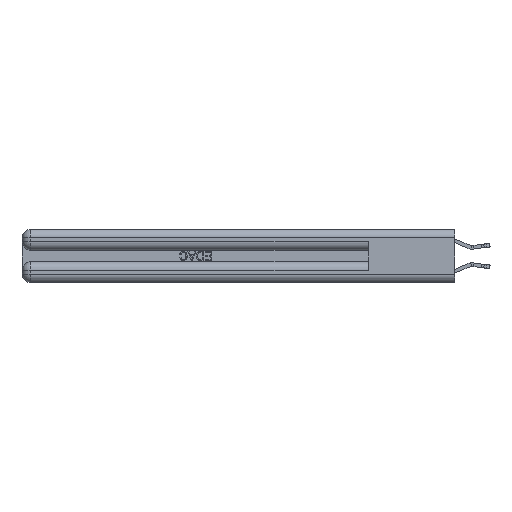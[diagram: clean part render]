
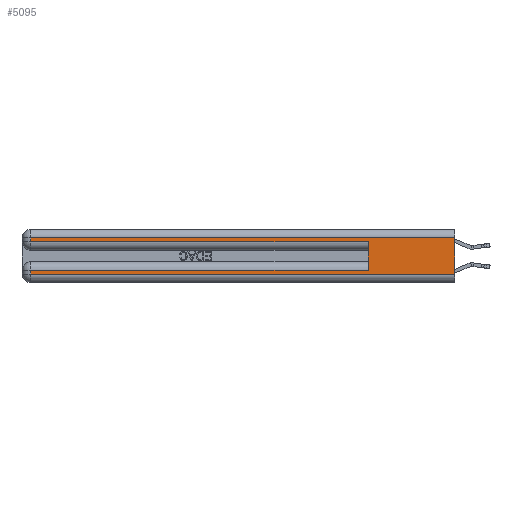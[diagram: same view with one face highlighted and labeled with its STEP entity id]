
A CAD part, left-side view. The second image highlights one B-rep face of the part: STEP entity #5095.
In plain terms, the highlighted planar face has unit normal (-1, 0, 0).
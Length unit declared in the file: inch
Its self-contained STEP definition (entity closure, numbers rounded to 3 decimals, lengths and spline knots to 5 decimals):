
#243 = ORIENTED_EDGE ( 'NONE', *, *, #14058, .T. ) ;
#817 = EDGE_CURVE ( 'NONE', #19369, #14251, #12594, .T. ) ;
#1171 = CARTESIAN_POINT ( 'NONE',  ( 0., 2.94, 0.31 ) ) ;
#3364 = ORIENTED_EDGE ( 'NONE', *, *, #25853, .T. ) ;
#3532 = VERTEX_POINT ( 'NONE', #23146 ) ;
#3618 = CARTESIAN_POINT ( 'NONE',  ( 0., 2.94, 0.085 ) ) ;
#4390 = DIRECTION ( 'NONE',  ( 0., -1., 0. ) ) ;
#4689 = DIRECTION ( 'NONE',  ( 0., 0., -1. ) ) ;
#5095 = ADVANCED_FACE ( 'NONE', ( #7560 ), #18042, .F. ) ;
#5847 = LINE ( 'NONE', #16023, #31068 ) ;
#6286 = EDGE_CURVE ( 'NONE', #14251, #9467, #25667, .T. ) ;
#6995 = VECTOR ( 'NONE', #9151, 39.37008 ) ;
#7011 = VERTEX_POINT ( 'NONE', #24917 ) ;
#7443 = EDGE_CURVE ( 'NONE', #19369, #24441, #17260, .T. ) ;
#7560 = FACE_OUTER_BOUND ( 'NONE', #12107, .T. ) ;
#8451 = CARTESIAN_POINT ( 'NONE',  ( 0., 0.6, 0.285 ) ) ;
#9151 = DIRECTION ( 'NONE',  ( 0., 0., 1. ) ) ;
#9343 = CARTESIAN_POINT ( 'NONE',  ( 0., 0., 0.37 ) ) ;
#9467 = VERTEX_POINT ( 'NONE', #26497 ) ;
#9583 = ORIENTED_EDGE ( 'NONE', *, *, #817, .T. ) ;
#10429 = DIRECTION ( 'NONE',  ( 0., 1., 0. ) ) ;
#11110 = AXIS2_PLACEMENT_3D ( 'NONE', #12486, #30689, #4689 ) ;
#11190 = DIRECTION ( 'NONE',  ( 0., 0., -1. ) ) ;
#12107 = EDGE_LOOP ( 'NONE', ( #27706, #17605, #17052, #243, #27524, #9583, #22350, #3364 ) ) ;
#12486 = CARTESIAN_POINT ( 'NONE',  ( 0., 0., 0.37 ) ) ;
#12594 = LINE ( 'NONE', #20213, #22159 ) ;
#12646 = CARTESIAN_POINT ( 'NONE',  ( 0., 2.94, 0.285 ) ) ;
#14058 = EDGE_CURVE ( 'NONE', #20935, #24441, #21503, .T. ) ;
#14251 = VERTEX_POINT ( 'NONE', #3618 ) ;
#14434 = DIRECTION ( 'NONE',  ( 0., 0., -1. ) ) ;
#15524 = CARTESIAN_POINT ( 'NONE',  ( 0., 2.94, 0.37 ) ) ;
#16023 = CARTESIAN_POINT ( 'NONE',  ( 0., 0., 0.31 ) ) ;
#17052 = ORIENTED_EDGE ( 'NONE', *, *, #31156, .T. ) ;
#17260 = LINE ( 'NONE', #26900, #6995 ) ;
#17605 = ORIENTED_EDGE ( 'NONE', *, *, #29903, .T. ) ;
#17768 = VECTOR ( 'NONE', #14434, 39.37008 ) ;
#18042 = PLANE ( 'NONE',  #11110 ) ;
#18788 = CARTESIAN_POINT ( 'NONE',  ( 0., 2.94, 0.37 ) ) ;
#19369 = VERTEX_POINT ( 'NONE', #31882 ) ;
#19452 = CARTESIAN_POINT ( 'NONE',  ( 0., 0., 0.06 ) ) ;
#19912 = EDGE_CURVE ( 'NONE', #7011, #3532, #22369, .T. ) ;
#20213 = CARTESIAN_POINT ( 'NONE',  ( 0., 0., 0.085 ) ) ;
#20935 = VERTEX_POINT ( 'NONE', #12646 ) ;
#21261 = VECTOR ( 'NONE', #31094, 39.37008 ) ;
#21503 = LINE ( 'NONE', #31761, #21261 ) ;
#21508 = LINE ( 'NONE', #18788, #31112 ) ;
#22046 = VECTOR ( 'NONE', #25817, 39.37008 ) ;
#22159 = VECTOR ( 'NONE', #32502, 39.37008 ) ;
#22350 = ORIENTED_EDGE ( 'NONE', *, *, #6286, .T. ) ;
#22369 = LINE ( 'NONE', #9343, #17768 ) ;
#23146 = CARTESIAN_POINT ( 'NONE',  ( 0., 0., 0.06 ) ) ;
#24441 = VERTEX_POINT ( 'NONE', #8451 ) ;
#24551 = VERTEX_POINT ( 'NONE', #1171 ) ;
#24917 = CARTESIAN_POINT ( 'NONE',  ( 0., 0., 0.31 ) ) ;
#25527 = VECTOR ( 'NONE', #4390, 39.37008 ) ;
#25667 = LINE ( 'NONE', #15524, #22046 ) ;
#25817 = DIRECTION ( 'NONE',  ( 0., 0., -1. ) ) ;
#25853 = EDGE_CURVE ( 'NONE', #9467, #3532, #27540, .T. ) ;
#26497 = CARTESIAN_POINT ( 'NONE',  ( 0., 2.94, 0.06 ) ) ;
#26900 = CARTESIAN_POINT ( 'NONE',  ( 0., 0.6, 0.145 ) ) ;
#27524 = ORIENTED_EDGE ( 'NONE', *, *, #7443, .F. ) ;
#27540 = LINE ( 'NONE', #19452, #25527 ) ;
#27706 = ORIENTED_EDGE ( 'NONE', *, *, #19912, .F. ) ;
#29903 = EDGE_CURVE ( 'NONE', #7011, #24551, #5847, .T. ) ;
#30689 = DIRECTION ( 'NONE',  ( 1., 0., 0. ) ) ;
#31068 = VECTOR ( 'NONE', #10429, 39.37008 ) ;
#31094 = DIRECTION ( 'NONE',  ( 0., -1., 0. ) ) ;
#31112 = VECTOR ( 'NONE', #11190, 39.37008 ) ;
#31156 = EDGE_CURVE ( 'NONE', #24551, #20935, #21508, .T. ) ;
#31761 = CARTESIAN_POINT ( 'NONE',  ( 0., 0., 0.285 ) ) ;
#31882 = CARTESIAN_POINT ( 'NONE',  ( 0., 0.6, 0.085 ) ) ;
#32502 = DIRECTION ( 'NONE',  ( 0., 1., 0. ) ) ;
